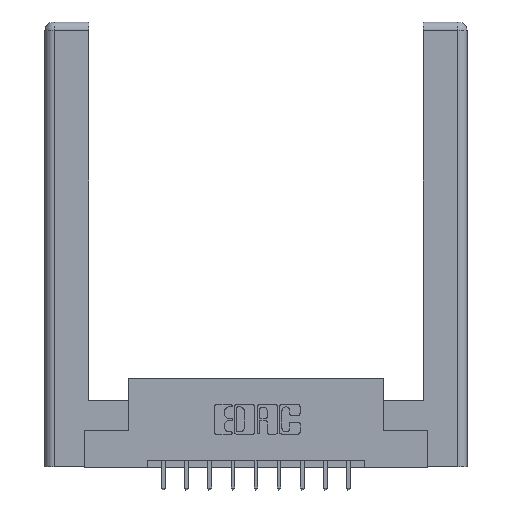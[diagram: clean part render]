
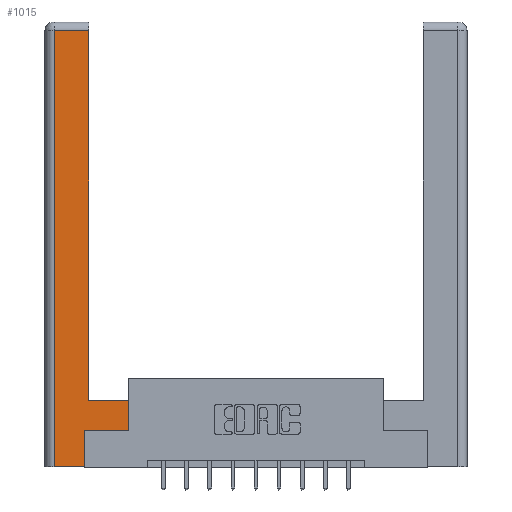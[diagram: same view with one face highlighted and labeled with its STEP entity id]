
A CAD part, top view. The second image highlights one B-rep face of the part: STEP entity #1015.
In plain terms, the highlighted planar face has unit normal (0, 0, 1).
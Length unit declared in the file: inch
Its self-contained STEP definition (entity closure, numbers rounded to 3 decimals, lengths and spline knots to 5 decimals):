
#331 = DIRECTION ( 'NONE',  ( 0., 0., -1. ) ) ;
#545 = LINE ( 'NONE', #3404, #5821 ) ;
#607 = LINE ( 'NONE', #7113, #4531 ) ;
#702 = EDGE_CURVE ( 'NONE', #7503, #2616, #2704, .T. ) ;
#895 = CARTESIAN_POINT ( 'NONE',  ( 0.265, 0., 0. ) ) ;
#1015 = ADVANCED_FACE ( 'NONE', ( #13240 ), #5830, .F. ) ;
#1278 = EDGE_CURVE ( 'NONE', #5828, #7503, #607, .T. ) ;
#1446 = CARTESIAN_POINT ( 'NONE',  ( 0.295, 3., 0. ) ) ;
#2289 = CARTESIAN_POINT ( 'NONE',  ( 0.295, 2.94, 0. ) ) ;
#2353 = DIRECTION ( 'NONE',  ( -1., 0., 0. ) ) ;
#2401 = ORIENTED_EDGE ( 'NONE', *, *, #3944, .T. ) ;
#2616 = VERTEX_POINT ( 'NONE', #895 ) ;
#2704 = LINE ( 'NONE', #4163, #4207 ) ;
#2930 = ORIENTED_EDGE ( 'NONE', *, *, #1278, .T. ) ;
#3009 = EDGE_CURVE ( 'NONE', #13860, #5828, #545, .T. ) ;
#3087 = VERTEX_POINT ( 'NONE', #5951 ) ;
#3404 = CARTESIAN_POINT ( 'NONE',  ( 0.0615, 2.94, 0. ) ) ;
#3549 = CARTESIAN_POINT ( 'NONE',  ( 0.265, 0.245, 0. ) ) ;
#3607 = ORIENTED_EDGE ( 'NONE', *, *, #702, .T. ) ;
#3807 = ORIENTED_EDGE ( 'NONE', *, *, #3009, .T. ) ;
#3944 = EDGE_CURVE ( 'NONE', #7543, #13860, #10436, .T. ) ;
#4163 = CARTESIAN_POINT ( 'NONE',  ( 0.265, 0., 0. ) ) ;
#4207 = VECTOR ( 'NONE', #4301, 39.37008 ) ;
#4301 = DIRECTION ( 'NONE',  ( 1., 0., 0. ) ) ;
#4531 = VECTOR ( 'NONE', #10354, 39.37008 ) ;
#4646 = CARTESIAN_POINT ( 'NONE',  ( 0., 0., 0. ) ) ;
#4680 = LINE ( 'NONE', #7127, #12026 ) ;
#5027 = DIRECTION ( 'NONE',  ( 1., 0., 0. ) ) ;
#5661 = DIRECTION ( 'NONE',  ( -1., 0., 0. ) ) ;
#5821 = VECTOR ( 'NONE', #2353, 39.37008 ) ;
#5828 = VERTEX_POINT ( 'NONE', #13487 ) ;
#5830 = PLANE ( 'NONE',  #8423 ) ;
#5873 = DIRECTION ( 'NONE',  ( 0., 1., 0. ) ) ;
#5880 = DIRECTION ( 'NONE',  ( -1., 0., 0. ) ) ;
#5951 = CARTESIAN_POINT ( 'NONE',  ( 0.565, 0.245, 0. ) ) ;
#5978 = ORIENTED_EDGE ( 'NONE', *, *, #8848, .T. ) ;
#6798 = VECTOR ( 'NONE', #8933, 39.37008 ) ;
#7113 = CARTESIAN_POINT ( 'NONE',  ( 0.0615, 0., 0. ) ) ;
#7127 = CARTESIAN_POINT ( 'NONE',  ( 0.565, 0.245, 0. ) ) ;
#7503 = VERTEX_POINT ( 'NONE', #9998 ) ;
#7518 = EDGE_CURVE ( 'NONE', #3087, #9829, #12203, .T. ) ;
#7543 = VERTEX_POINT ( 'NONE', #7732 ) ;
#7592 = EDGE_CURVE ( 'NONE', #12484, #3087, #4680, .T. ) ;
#7732 = CARTESIAN_POINT ( 'NONE',  ( 0.295, 0.45, 0. ) ) ;
#7749 = CARTESIAN_POINT ( 'NONE',  ( 0.295, 0.45, 0. ) ) ;
#7964 = LINE ( 'NONE', #7749, #9940 ) ;
#8423 = AXIS2_PLACEMENT_3D ( 'NONE', #4646, #331, #5880 ) ;
#8518 = VECTOR ( 'NONE', #12012, 39.37008 ) ;
#8798 = CARTESIAN_POINT ( 'NONE',  ( 0.565, 0.45, 0. ) ) ;
#8848 = EDGE_CURVE ( 'NONE', #2616, #12484, #10960, .T. ) ;
#8933 = DIRECTION ( 'NONE',  ( 0., 1., 0. ) ) ;
#9102 = EDGE_LOOP ( 'NONE', ( #2401, #3807, #2930, #3607, #5978, #9769, #13534, #11675 ) ) ;
#9270 = VECTOR ( 'NONE', #5873, 39.37008 ) ;
#9769 = ORIENTED_EDGE ( 'NONE', *, *, #7592, .T. ) ;
#9772 = CARTESIAN_POINT ( 'NONE',  ( 0.565, 0.45, 0. ) ) ;
#9829 = VERTEX_POINT ( 'NONE', #9772 ) ;
#9940 = VECTOR ( 'NONE', #5661, 39.37008 ) ;
#9998 = CARTESIAN_POINT ( 'NONE',  ( 0.0615, 0., 0. ) ) ;
#10354 = DIRECTION ( 'NONE',  ( 0., -1., 0. ) ) ;
#10436 = LINE ( 'NONE', #1446, #9270 ) ;
#10960 = LINE ( 'NONE', #3549, #6798 ) ;
#11549 = EDGE_CURVE ( 'NONE', #9829, #7543, #7964, .T. ) ;
#11675 = ORIENTED_EDGE ( 'NONE', *, *, #11549, .T. ) ;
#12012 = DIRECTION ( 'NONE',  ( 0., 1., 0. ) ) ;
#12026 = VECTOR ( 'NONE', #5027, 39.37008 ) ;
#12203 = LINE ( 'NONE', #8798, #8518 ) ;
#12484 = VERTEX_POINT ( 'NONE', #13080 ) ;
#13080 = CARTESIAN_POINT ( 'NONE',  ( 0.265, 0.245, 0. ) ) ;
#13240 = FACE_OUTER_BOUND ( 'NONE', #9102, .T. ) ;
#13487 = CARTESIAN_POINT ( 'NONE',  ( 0.0615, 2.94, 0. ) ) ;
#13534 = ORIENTED_EDGE ( 'NONE', *, *, #7518, .T. ) ;
#13860 = VERTEX_POINT ( 'NONE', #2289 ) ;
